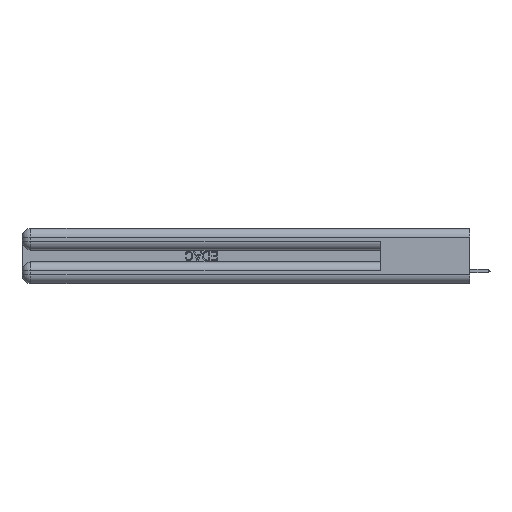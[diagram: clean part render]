
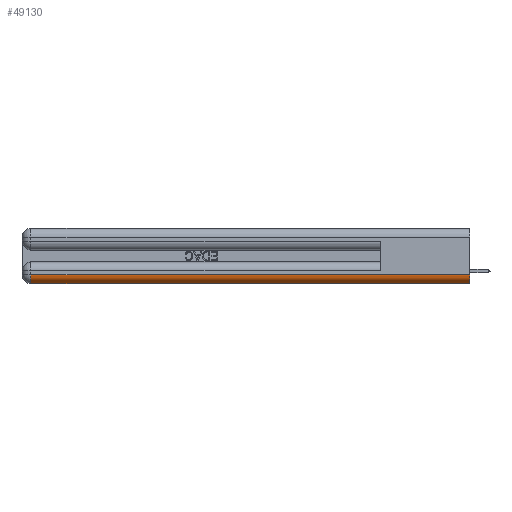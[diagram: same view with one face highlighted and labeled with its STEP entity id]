
A CAD part, left-side view. The second image highlights one B-rep face of the part: STEP entity #49130.
In plain terms, the highlighted cylindrical face has radius 1.524 mm (diameter 3.048 mm), a partial arc.
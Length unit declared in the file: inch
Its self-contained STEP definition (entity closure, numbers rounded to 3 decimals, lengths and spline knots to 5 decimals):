
#722 = CIRCLE ( 'NONE', #26697, 0.06 ) ;
#2357 = ORIENTED_EDGE ( 'NONE', *, *, #45033, .F. ) ;
#3880 = CARTESIAN_POINT ( 'NONE',  ( 0., 0., 0.06 ) ) ;
#4387 = DIRECTION ( 'NONE',  ( 0., -1., 0. ) ) ;
#4396 = DIRECTION ( 'NONE',  ( 0., 1., 0. ) ) ;
#4729 = ORIENTED_EDGE ( 'NONE', *, *, #30805, .F. ) ;
#8133 = EDGE_LOOP ( 'NONE', ( #4729, #2357, #43380, #49855 ) ) ;
#11375 = DIRECTION ( 'NONE',  ( 0., 0., 1. ) ) ;
#12780 = VERTEX_POINT ( 'NONE', #3880 ) ;
#14453 = CARTESIAN_POINT ( 'NONE',  ( 0.06, 2.94, 0. ) ) ;
#17247 = VERTEX_POINT ( 'NONE', #39931 ) ;
#18512 = LINE ( 'NONE', #39202, #41380 ) ;
#20717 = VERTEX_POINT ( 'NONE', #21938 ) ;
#21126 = CARTESIAN_POINT ( 'NONE',  ( 0.06, 2.94, 0.06 ) ) ;
#21938 = CARTESIAN_POINT ( 'NONE',  ( 0., 2.94, 0.06 ) ) ;
#21992 = DIRECTION ( 'NONE',  ( 0., 0., 1. ) ) ;
#26211 = CARTESIAN_POINT ( 'NONE',  ( 0.06, 0., 0.06 ) ) ;
#26697 = AXIS2_PLACEMENT_3D ( 'NONE', #21126, #45581, #21992 ) ;
#26700 = DIRECTION ( 'NONE',  ( 0., 1., 0. ) ) ;
#28149 = VERTEX_POINT ( 'NONE', #14453 ) ;
#29829 = DIRECTION ( 'NONE',  ( 0., 0., 1. ) ) ;
#30805 = EDGE_CURVE ( 'NONE', #12780, #17247, #34417, .T. ) ;
#31569 = CYLINDRICAL_SURFACE ( 'NONE', #35248, 0.06 ) ;
#34417 = CIRCLE ( 'NONE', #46770, 0.06 ) ;
#35248 = AXIS2_PLACEMENT_3D ( 'NONE', #46189, #26700, #11375 ) ;
#36536 = FACE_OUTER_BOUND ( 'NONE', #8133, .T. ) ;
#39202 = CARTESIAN_POINT ( 'NONE',  ( 0., 0., 0.06 ) ) ;
#39931 = CARTESIAN_POINT ( 'NONE',  ( 0.06, 0., 0. ) ) ;
#41380 = VECTOR ( 'NONE', #4387, 39.37008 ) ;
#41944 = EDGE_CURVE ( 'NONE', #17247, #28149, #48397, .T. ) ;
#42870 = VECTOR ( 'NONE', #4396, 39.37008 ) ;
#43380 = ORIENTED_EDGE ( 'NONE', *, *, #50197, .F. ) ;
#45033 = EDGE_CURVE ( 'NONE', #20717, #12780, #18512, .T. ) ;
#45581 = DIRECTION ( 'NONE',  ( 0., 1., 0. ) ) ;
#46189 = CARTESIAN_POINT ( 'NONE',  ( 0.06, 0., 0.06 ) ) ;
#46770 = AXIS2_PLACEMENT_3D ( 'NONE', #26211, #49633, #29829 ) ;
#48146 = CARTESIAN_POINT ( 'NONE',  ( 0.06, 3., 0. ) ) ;
#48397 = LINE ( 'NONE', #48146, #42870 ) ;
#49130 = ADVANCED_FACE ( 'NONE', ( #36536 ), #31569, .T. ) ;
#49633 = DIRECTION ( 'NONE',  ( 0., -1., 0. ) ) ;
#49855 = ORIENTED_EDGE ( 'NONE', *, *, #41944, .F. ) ;
#50197 = EDGE_CURVE ( 'NONE', #28149, #20717, #722, .T. ) ;
